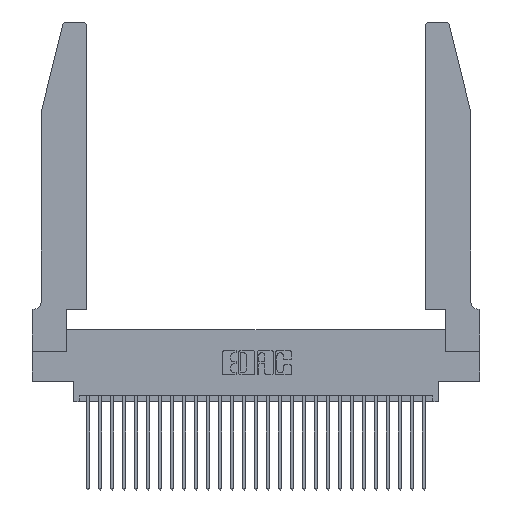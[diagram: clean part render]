
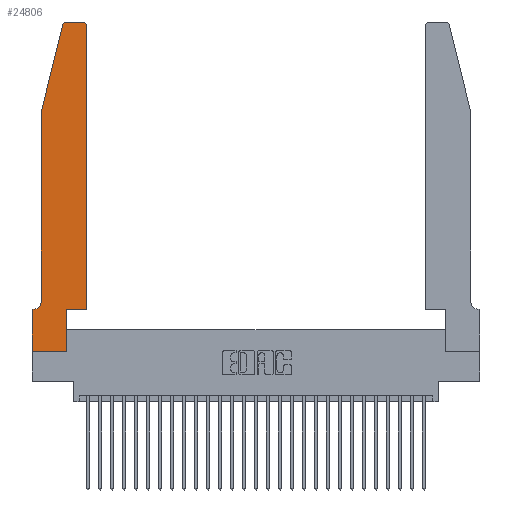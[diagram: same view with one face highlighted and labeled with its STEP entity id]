
A CAD part, top view. The second image highlights one B-rep face of the part: STEP entity #24806.
In plain terms, the highlighted planar face has unit normal (0, 0, 1).
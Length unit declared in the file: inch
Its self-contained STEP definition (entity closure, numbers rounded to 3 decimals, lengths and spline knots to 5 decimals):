
#576 = VERTEX_POINT ( 'NONE', #22450 ) ;
#1354 = EDGE_CURVE ( 'NONE', #21691, #6707, #19102, .T. ) ;
#1612 = VERTEX_POINT ( 'NONE', #3034 ) ;
#1682 = LINE ( 'NONE', #9600, #11699 ) ;
#1876 = AXIS2_PLACEMENT_3D ( 'NONE', #12501, #28277, #14770 ) ;
#2285 = CARTESIAN_POINT ( 'NONE',  ( 0.284, 2.72, 0.37 ) ) ;
#3018 = DIRECTION ( 'NONE',  ( 0., -1., 0. ) ) ;
#3034 = CARTESIAN_POINT ( 'NONE',  ( 0., 0.35, 0.37 ) ) ;
#3687 = DIRECTION ( 'NONE',  ( 1., 0., 0. ) ) ;
#4608 = DIRECTION ( 'NONE',  ( 1., 0., 0. ) ) ;
#4691 = EDGE_CURVE ( 'NONE', #576, #17016, #10867, .T. ) ;
#5360 = EDGE_CURVE ( 'NONE', #14086, #21299, #19682, .T. ) ;
#5707 = CARTESIAN_POINT ( 'NONE',  ( 0.0755, 2., 0.37 ) ) ;
#5805 = DIRECTION ( 'NONE',  ( -0.239, -0.971, 0. ) ) ;
#5986 = CARTESIAN_POINT ( 'NONE',  ( 0., 0., 0.37 ) ) ;
#6248 = CARTESIAN_POINT ( 'NONE',  ( 0.0755, 0.42, 0.37 ) ) ;
#6370 = EDGE_CURVE ( 'NONE', #8661, #22537, #19624, .T. ) ;
#6379 = LINE ( 'NONE', #6760, #23072 ) ;
#6397 = ORIENTED_EDGE ( 'NONE', *, *, #5360, .T. ) ;
#6707 = VERTEX_POINT ( 'NONE', #27446 ) ;
#6760 = CARTESIAN_POINT ( 'NONE',  ( 0.2865, 0.35, 0.37 ) ) ;
#7072 = DIRECTION ( 'NONE',  ( 1., 0., 0. ) ) ;
#7166 = VECTOR ( 'NONE', #22766, 39.37008 ) ;
#7497 = CARTESIAN_POINT ( 'NONE',  ( 0.0755, 2., 0.37 ) ) ;
#7524 = VECTOR ( 'NONE', #3687, 39.37008 ) ;
#7976 = VECTOR ( 'NONE', #20534, 39.37008 ) ;
#8129 = CARTESIAN_POINT ( 'NONE',  ( 0.284, 2.75, 0.37 ) ) ;
#8661 = VERTEX_POINT ( 'NONE', #11962 ) ;
#9209 = ORIENTED_EDGE ( 'NONE', *, *, #13703, .T. ) ;
#9410 = ORIENTED_EDGE ( 'NONE', *, *, #23279, .T. ) ;
#9456 = VECTOR ( 'NONE', #26819, 39.37008 ) ;
#9600 = CARTESIAN_POINT ( 'NONE',  ( 0., 0., 0.37 ) ) ;
#10173 = VERTEX_POINT ( 'NONE', #5707 ) ;
#10632 = DIRECTION ( 'NONE',  ( 0., 1., 0. ) ) ;
#10867 = LINE ( 'NONE', #22265, #7976 ) ;
#11230 = CIRCLE ( 'NONE', #1876, 0.07 ) ;
#11528 = EDGE_CURVE ( 'NONE', #12413, #24260, #11230, .T. ) ;
#11699 = VECTOR ( 'NONE', #11907, 39.37008 ) ;
#11907 = DIRECTION ( 'NONE',  ( 0., -1., 0. ) ) ;
#11962 = CARTESIAN_POINT ( 'NONE',  ( 0., 0., 0.37 ) ) ;
#12288 = AXIS2_PLACEMENT_3D ( 'NONE', #16099, #20683, #7072 ) ;
#12413 = VERTEX_POINT ( 'NONE', #6248 ) ;
#12501 = CARTESIAN_POINT ( 'NONE',  ( 0.0055, 0.42, 0.37 ) ) ;
#13226 = LINE ( 'NONE', #27156, #7166 ) ;
#13359 = DIRECTION ( 'NONE',  ( 1., 0., 0. ) ) ;
#13382 = DIRECTION ( 'NONE',  ( 0., 0., 1. ) ) ;
#13554 = CARTESIAN_POINT ( 'NONE',  ( 0.4205, 2.72, 0.37 ) ) ;
#13703 = EDGE_CURVE ( 'NONE', #24260, #1612, #13226, .T. ) ;
#14086 = VERTEX_POINT ( 'NONE', #8129 ) ;
#14088 = LINE ( 'NONE', #22326, #9456 ) ;
#14770 = DIRECTION ( 'NONE',  ( -1., 0., 0. ) ) ;
#15290 = EDGE_CURVE ( 'NONE', #17016, #21691, #26908, .T. ) ;
#15390 = DIRECTION ( 'NONE',  ( 0., 1., 0. ) ) ;
#15653 = EDGE_CURVE ( 'NONE', #1612, #8661, #1682, .T. ) ;
#15932 = CARTESIAN_POINT ( 'NONE',  ( 0.0055, 0.35, 0.37 ) ) ;
#16099 = CARTESIAN_POINT ( 'NONE',  ( 0., 0.35, 0.37 ) ) ;
#16761 = CARTESIAN_POINT ( 'NONE',  ( 0.2865, 0., 0.37 ) ) ;
#16896 = ORIENTED_EDGE ( 'NONE', *, *, #15290, .T. ) ;
#17016 = VERTEX_POINT ( 'NONE', #21541 ) ;
#17134 = VECTOR ( 'NONE', #5805, 39.37008 ) ;
#17203 = AXIS2_PLACEMENT_3D ( 'NONE', #2285, #18228, #4608 ) ;
#17449 = LINE ( 'NONE', #23958, #17134 ) ;
#17499 = EDGE_LOOP ( 'NONE', ( #24535, #6397, #9410, #21501, #21524, #9209, #18997, #24523, #27368, #18078, #16896, #24692 ) ) ;
#17795 = AXIS2_PLACEMENT_3D ( 'NONE', #13554, #13382, #13359 ) ;
#18078 = ORIENTED_EDGE ( 'NONE', *, *, #4691, .T. ) ;
#18228 = DIRECTION ( 'NONE',  ( 0., 0., 1. ) ) ;
#18355 = EDGE_CURVE ( 'NONE', #22537, #576, #6379, .T. ) ;
#18410 = PLANE ( 'NONE',  #12288 ) ;
#18997 = ORIENTED_EDGE ( 'NONE', *, *, #15653, .T. ) ;
#19102 = CIRCLE ( 'NONE', #17795, 0.03 ) ;
#19147 = CARTESIAN_POINT ( 'NONE',  ( 0.25487, 2.72718, 0.37 ) ) ;
#19164 = VECTOR ( 'NONE', #3018, 39.37008 ) ;
#19624 = LINE ( 'NONE', #5986, #7524 ) ;
#19682 = CIRCLE ( 'NONE', #17203, 0.03 ) ;
#19874 = LINE ( 'NONE', #7497, #19164 ) ;
#20534 = DIRECTION ( 'NONE',  ( 1., 0., 0. ) ) ;
#20683 = DIRECTION ( 'NONE',  ( 0., 0., 1. ) ) ;
#20994 = EDGE_CURVE ( 'NONE', #6707, #14086, #14088, .T. ) ;
#21299 = VERTEX_POINT ( 'NONE', #19147 ) ;
#21501 = ORIENTED_EDGE ( 'NONE', *, *, #25517, .T. ) ;
#21524 = ORIENTED_EDGE ( 'NONE', *, *, #11528, .T. ) ;
#21541 = CARTESIAN_POINT ( 'NONE',  ( 0.4505, 0.35, 0.37 ) ) ;
#21649 = VECTOR ( 'NONE', #10632, 39.37008 ) ;
#21691 = VERTEX_POINT ( 'NONE', #27179 ) ;
#21933 = CARTESIAN_POINT ( 'NONE',  ( 0.4505, 0.35, 0.37 ) ) ;
#22265 = CARTESIAN_POINT ( 'NONE',  ( 0.4505, 0.35, 0.37 ) ) ;
#22326 = CARTESIAN_POINT ( 'NONE',  ( 0.2605, 2.75, 0.37 ) ) ;
#22450 = CARTESIAN_POINT ( 'NONE',  ( 0.2865, 0.35, 0.37 ) ) ;
#22537 = VERTEX_POINT ( 'NONE', #16761 ) ;
#22766 = DIRECTION ( 'NONE',  ( -1., 0., 0. ) ) ;
#23072 = VECTOR ( 'NONE', #15390, 39.37008 ) ;
#23279 = EDGE_CURVE ( 'NONE', #21299, #10173, #17449, .T. ) ;
#23958 = CARTESIAN_POINT ( 'NONE',  ( 0.0755, 2., 0.37 ) ) ;
#24260 = VERTEX_POINT ( 'NONE', #15932 ) ;
#24523 = ORIENTED_EDGE ( 'NONE', *, *, #6370, .T. ) ;
#24535 = ORIENTED_EDGE ( 'NONE', *, *, #20994, .T. ) ;
#24692 = ORIENTED_EDGE ( 'NONE', *, *, #1354, .T. ) ;
#24806 = ADVANCED_FACE ( 'NONE', ( #25544 ), #18410, .T. ) ;
#25517 = EDGE_CURVE ( 'NONE', #10173, #12413, #19874, .T. ) ;
#25544 = FACE_OUTER_BOUND ( 'NONE', #17499, .T. ) ;
#26819 = DIRECTION ( 'NONE',  ( -1., 0., 0. ) ) ;
#26908 = LINE ( 'NONE', #21933, #21649 ) ;
#27156 = CARTESIAN_POINT ( 'NONE',  ( 0.0755, 0.35, 0.37 ) ) ;
#27179 = CARTESIAN_POINT ( 'NONE',  ( 0.4505, 2.72, 0.37 ) ) ;
#27368 = ORIENTED_EDGE ( 'NONE', *, *, #18355, .T. ) ;
#27446 = CARTESIAN_POINT ( 'NONE',  ( 0.4205, 2.75, 0.37 ) ) ;
#28277 = DIRECTION ( 'NONE',  ( 0., 0., -1. ) ) ;
